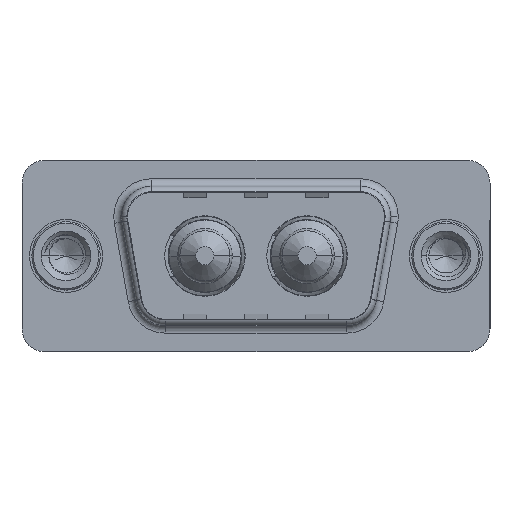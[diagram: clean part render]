
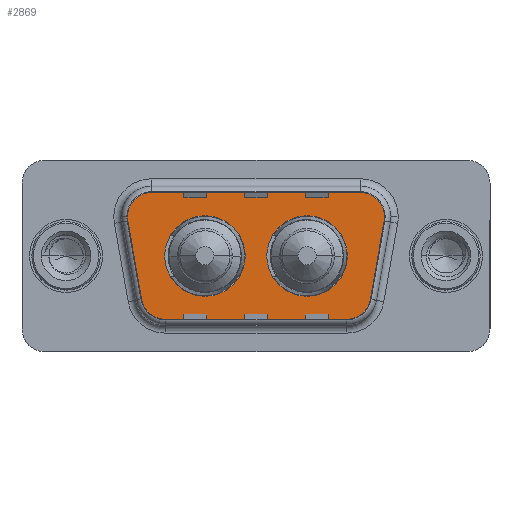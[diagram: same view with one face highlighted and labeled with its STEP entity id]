
A CAD part, top view. The second image highlights one B-rep face of the part: STEP entity #2869.
In plain terms, the highlighted planar face has unit normal (0, 0, 1).
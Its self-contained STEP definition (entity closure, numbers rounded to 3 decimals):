
#3 = EDGE_CURVE ( 'NONE', #1639, #10621, #3431, .T. ) ;
#263 = DIRECTION ( 'NONE',  ( 0., 0., 1. ) ) ;
#338 = VERTEX_POINT ( 'NONE', #4252 ) ;
#343 = VECTOR ( 'NONE', #7954, 1000. ) ;
#413 = DIRECTION ( 'NONE',  ( 0., 0., 1. ) ) ;
#481 = EDGE_CURVE ( 'NONE', #12034, #1639, #5226, .T. ) ;
#691 = AXIS2_PLACEMENT_3D ( 'NONE', #9078, #2129, #10248 ) ;
#702 = AXIS2_PLACEMENT_3D ( 'NONE', #4544, #10212, #12895 ) ;
#726 = VERTEX_POINT ( 'NONE', #5584 ) ;
#854 = CARTESIAN_POINT ( 'NONE',  ( 5.436, 4.9, 0. ) ) ;
#1034 = AXIS2_PLACEMENT_3D ( 'NONE', #2639, #2629, #2734 ) ;
#1326 = VECTOR ( 'NONE', #4335, 1000. ) ;
#1425 = EDGE_CURVE ( 'NONE', #338, #12034, #13245, .T. ) ;
#1639 = VERTEX_POINT ( 'NONE', #4064 ) ;
#1989 = CIRCLE ( 'NONE', #14089, 2.65 ) ;
#2129 = DIRECTION ( 'NONE',  ( 0., 0., 1. ) ) ;
#2359 = ORIENTED_EDGE ( 'NONE', *, *, #1425, .T. ) ;
#2419 = DIRECTION ( 'NONE',  ( 0., 0., 1. ) ) ;
#2462 = CARTESIAN_POINT ( 'NONE',  ( 4.489, -3.247, 0. ) ) ;
#2510 = ORIENTED_EDGE ( 'NONE', *, *, #6466, .T. ) ;
#2575 = DIRECTION ( 'NONE',  ( -1., 0., 0. ) ) ;
#2629 = DIRECTION ( 'NONE',  ( 0., 0., 1. ) ) ;
#2639 = CARTESIAN_POINT ( 'NONE',  ( 18.541, -2.9, 0. ) ) ;
#2734 = DIRECTION ( 'NONE',  ( 1., 0., 0. ) ) ;
#2757 = EDGE_CURVE ( 'NONE', #5797, #14269, #12506, .T. ) ;
#2869 = ADVANCED_FACE ( 'NONE', ( #14126, #8265, #11409 ), #9631, .T. ) ;
#3090 = DIRECTION ( 'NONE',  ( 1., 0., 0. ) ) ;
#3185 = CARTESIAN_POINT ( 'NONE',  ( 5.436, 4.9, 0. ) ) ;
#3310 = CARTESIAN_POINT ( 'NONE',  ( 19.564, 4.9, 0. ) ) ;
#3336 = ORIENTED_EDGE ( 'NONE', *, *, #3, .T. ) ;
#3377 = LINE ( 'NONE', #13365, #12319 ) ;
#3431 = LINE ( 'NONE', #3630, #343 ) ;
#3456 = AXIS2_PLACEMENT_3D ( 'NONE', #7358, #413, #8545 ) ;
#3630 = CARTESIAN_POINT ( 'NONE',  ( 6.459, -4.9, 0. ) ) ;
#4040 = DIRECTION ( 'NONE',  ( 0., 0., 1. ) ) ;
#4064 = CARTESIAN_POINT ( 'NONE',  ( 6.459, -4.9, 0. ) ) ;
#4252 = CARTESIAN_POINT ( 'NONE',  ( 3.466, 2.553, 0. ) ) ;
#4335 = DIRECTION ( 'NONE',  ( -1., 0., 0. ) ) ;
#4396 = EDGE_LOOP ( 'NONE', ( #8418, #7889 ) ) ;
#4544 = CARTESIAN_POINT ( 'NONE',  ( 18.541, -2.9, 0. ) ) ;
#4767 = LINE ( 'NONE', #3185, #1326 ) ;
#4785 = EDGE_CURVE ( 'NONE', #14269, #5797, #1989, .T. ) ;
#4939 = ORIENTED_EDGE ( 'NONE', *, *, #481, .T. ) ;
#5137 = EDGE_CURVE ( 'NONE', #10621, #14450, #8710, .T. ) ;
#5226 = CIRCLE ( 'NONE', #7960, 2. ) ;
#5584 = CARTESIAN_POINT ( 'NONE',  ( 6.49, 0., 0. ) ) ;
#5695 = EDGE_CURVE ( 'NONE', #726, #7075, #8697, .T. ) ;
#5744 = EDGE_CURVE ( 'NONE', #7075, #726, #8308, .T. ) ;
#5797 = VERTEX_POINT ( 'NONE', #10613 ) ;
#6034 = DIRECTION ( 'NONE',  ( 0.174, -0.985, 0. ) ) ;
#6069 = CARTESIAN_POINT ( 'NONE',  ( 9.14, 0., 0. ) ) ;
#6414 = AXIS2_PLACEMENT_3D ( 'NONE', #12383, #12574, #12854 ) ;
#6454 = CARTESIAN_POINT ( 'NONE',  ( 9.14, 0., 0. ) ) ;
#6466 = EDGE_CURVE ( 'NONE', #13884, #12029, #9205, .T. ) ;
#6539 = EDGE_LOOP ( 'NONE', ( #6984, #10601 ) ) ;
#6728 = AXIS2_PLACEMENT_3D ( 'NONE', #7200, #263, #8386 ) ;
#6772 = CIRCLE ( 'NONE', #691, 2. ) ;
#6947 = CARTESIAN_POINT ( 'NONE',  ( 20.511, -3.247, 0. ) ) ;
#6960 = EDGE_CURVE ( 'NONE', #14450, #13884, #3377, .T. ) ;
#6984 = ORIENTED_EDGE ( 'NONE', *, *, #5744, .F. ) ;
#6990 = ORIENTED_EDGE ( 'NONE', *, *, #13438, .T. ) ;
#7075 = VERTEX_POINT ( 'NONE', #7690 ) ;
#7200 = CARTESIAN_POINT ( 'NONE',  ( 5.436, 2.9, 0. ) ) ;
#7358 = CARTESIAN_POINT ( 'NONE',  ( 19.564, 2.9, 0. ) ) ;
#7401 = CARTESIAN_POINT ( 'NONE',  ( 21.534, 2.553, 0. ) ) ;
#7458 = ORIENTED_EDGE ( 'NONE', *, *, #13747, .T. ) ;
#7690 = CARTESIAN_POINT ( 'NONE',  ( 11.79, 0., 0. ) ) ;
#7889 = ORIENTED_EDGE ( 'NONE', *, *, #4785, .F. ) ;
#7950 = ORIENTED_EDGE ( 'NONE', *, *, #6960, .T. ) ;
#7954 = DIRECTION ( 'NONE',  ( 1., 0., 0. ) ) ;
#7960 = AXIS2_PLACEMENT_3D ( 'NONE', #14864, #8283, #2575 ) ;
#8205 = AXIS2_PLACEMENT_3D ( 'NONE', #6454, #4040, #3090 ) ;
#8265 = FACE_BOUND ( 'NONE', #6539, .T. ) ;
#8283 = DIRECTION ( 'NONE',  ( 0., 0., 1. ) ) ;
#8308 = CIRCLE ( 'NONE', #11385, 2.65 ) ;
#8386 = DIRECTION ( 'NONE',  ( 1., 0., 0. ) ) ;
#8418 = ORIENTED_EDGE ( 'NONE', *, *, #2757, .F. ) ;
#8490 = CARTESIAN_POINT ( 'NONE',  ( 15.86, 0., 0. ) ) ;
#8545 = DIRECTION ( 'NONE',  ( -1., 0., 0. ) ) ;
#8697 = CIRCLE ( 'NONE', #8205, 2.65 ) ;
#8710 = CIRCLE ( 'NONE', #1034, 2. ) ;
#8739 = VERTEX_POINT ( 'NONE', #854 ) ;
#9078 = CARTESIAN_POINT ( 'NONE',  ( 19.564, 2.9, 0. ) ) ;
#9107 = CARTESIAN_POINT ( 'NONE',  ( 18.541, -4.9, 0. ) ) ;
#9205 = CIRCLE ( 'NONE', #3456, 2. ) ;
#9298 = ORIENTED_EDGE ( 'NONE', *, *, #5137, .T. ) ;
#9414 = DIRECTION ( 'NONE',  ( 0., 0., 1. ) ) ;
#9631 = PLANE ( 'NONE',  #702 ) ;
#9761 = VECTOR ( 'NONE', #6034, 1000. ) ;
#9884 = DIRECTION ( 'NONE',  ( 1., 0., 0. ) ) ;
#10206 = EDGE_CURVE ( 'NONE', #12029, #11292, #6772, .T. ) ;
#10212 = DIRECTION ( 'NONE',  ( 0., 0., 1. ) ) ;
#10213 = ORIENTED_EDGE ( 'NONE', *, *, #10206, .T. ) ;
#10248 = DIRECTION ( 'NONE',  ( -1., 0., 0. ) ) ;
#10601 = ORIENTED_EDGE ( 'NONE', *, *, #5695, .F. ) ;
#10602 = CARTESIAN_POINT ( 'NONE',  ( 21.564, 2.9, 0. ) ) ;
#10613 = CARTESIAN_POINT ( 'NONE',  ( 18.51, 0., 0. ) ) ;
#10621 = VERTEX_POINT ( 'NONE', #9107 ) ;
#11115 = EDGE_LOOP ( 'NONE', ( #9298, #7950, #2510, #10213, #6990, #7458, #2359, #4939, #3336 ) ) ;
#11129 = CARTESIAN_POINT ( 'NONE',  ( 13.21, 0., 0. ) ) ;
#11292 = VERTEX_POINT ( 'NONE', #3310 ) ;
#11385 = AXIS2_PLACEMENT_3D ( 'NONE', #6069, #9414, #9884 ) ;
#11409 = FACE_OUTER_BOUND ( 'NONE', #11115, .T. ) ;
#12029 = VERTEX_POINT ( 'NONE', #10602 ) ;
#12034 = VERTEX_POINT ( 'NONE', #2462 ) ;
#12319 = VECTOR ( 'NONE', #14535, 1000. ) ;
#12383 = CARTESIAN_POINT ( 'NONE',  ( 15.86, 0., 0. ) ) ;
#12506 = CIRCLE ( 'NONE', #6414, 2.65 ) ;
#12574 = DIRECTION ( 'NONE',  ( 0., 0., 1. ) ) ;
#12654 = CARTESIAN_POINT ( 'NONE',  ( 3.466, 2.553, 0. ) ) ;
#12829 = DIRECTION ( 'NONE',  ( 1., 0., 0. ) ) ;
#12854 = DIRECTION ( 'NONE',  ( 1., 0., 0. ) ) ;
#12895 = DIRECTION ( 'NONE',  ( 1., 0., 0. ) ) ;
#13245 = LINE ( 'NONE', #12654, #9761 ) ;
#13365 = CARTESIAN_POINT ( 'NONE',  ( 21.534, 2.553, 0. ) ) ;
#13438 = EDGE_CURVE ( 'NONE', #11292, #8739, #4767, .T. ) ;
#13747 = EDGE_CURVE ( 'NONE', #8739, #338, #13903, .T. ) ;
#13884 = VERTEX_POINT ( 'NONE', #7401 ) ;
#13903 = CIRCLE ( 'NONE', #6728, 2. ) ;
#14089 = AXIS2_PLACEMENT_3D ( 'NONE', #8490, #2419, #12829 ) ;
#14126 = FACE_BOUND ( 'NONE', #4396, .T. ) ;
#14269 = VERTEX_POINT ( 'NONE', #11129 ) ;
#14450 = VERTEX_POINT ( 'NONE', #6947 ) ;
#14535 = DIRECTION ( 'NONE',  ( 0.174, 0.985, 0. ) ) ;
#14864 = CARTESIAN_POINT ( 'NONE',  ( 6.459, -2.9, 0. ) ) ;
